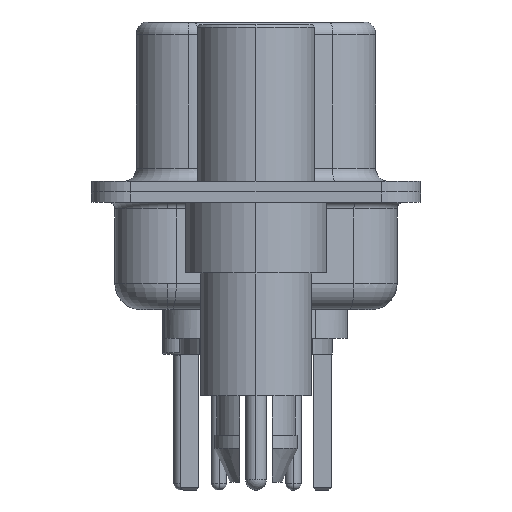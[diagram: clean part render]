
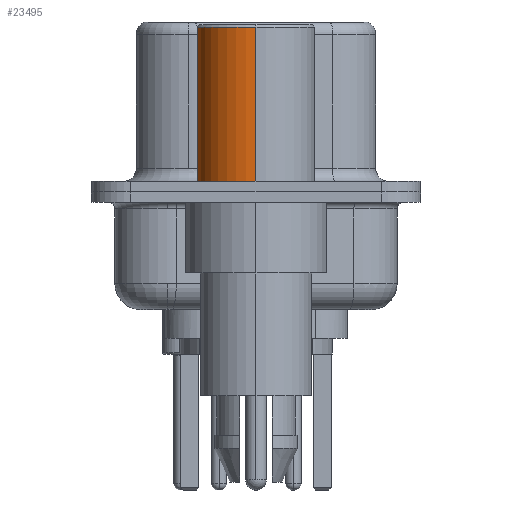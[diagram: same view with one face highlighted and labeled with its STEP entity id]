
A CAD part, left-side view. The second image highlights one B-rep face of the part: STEP entity #23495.
In plain terms, the highlighted cylindrical face has radius 2.25 mm (diameter 4.5 mm), a partial arc.
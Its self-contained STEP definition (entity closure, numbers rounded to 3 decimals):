
#470 = FACE_OUTER_BOUND ( 'NONE', #22428, .T. ) ;
#555 = DIRECTION ( 'NONE',  ( 0., 0., 1. ) ) ;
#798 = CARTESIAN_POINT ( 'NONE',  ( 0., 0., 0.4 ) ) ;
#839 = DIRECTION ( 'NONE',  ( 1., 0., 0. ) ) ;
#1047 = LINE ( 'NONE', #11443, #3647 ) ;
#1614 = CIRCLE ( 'NONE', #9624, 2.25 ) ;
#1945 = VECTOR ( 'NONE', #555, 1000. ) ;
#2211 = ORIENTED_EDGE ( 'NONE', *, *, #14536, .T. ) ;
#2398 = EDGE_CURVE ( 'NONE', #5247, #7590, #1614, .T. ) ;
#3647 = VECTOR ( 'NONE', #21915, 1000. ) ;
#3796 = ORIENTED_EDGE ( 'NONE', *, *, #12937, .F. ) ;
#4048 = AXIS2_PLACEMENT_3D ( 'NONE', #8427, #14633, #8522 ) ;
#5247 = VERTEX_POINT ( 'NONE', #15278 ) ;
#5337 = CYLINDRICAL_SURFACE ( 'NONE', #4048, 2.25 ) ;
#7590 = VERTEX_POINT ( 'NONE', #15728 ) ;
#7631 = CARTESIAN_POINT ( 'NONE',  ( -2.25, 0., 0.4 ) ) ;
#7761 = LINE ( 'NONE', #19326, #1945 ) ;
#8427 = CARTESIAN_POINT ( 'NONE',  ( 0., 0., 0.581 ) ) ;
#8464 = VERTEX_POINT ( 'NONE', #18188 ) ;
#8522 = DIRECTION ( 'NONE',  ( 1., 0., 0. ) ) ;
#9273 = ORIENTED_EDGE ( 'NONE', *, *, #2398, .F. ) ;
#9369 = VERTEX_POINT ( 'NONE', #7631 ) ;
#9624 = AXIS2_PLACEMENT_3D ( 'NONE', #15163, #23126, #839 ) ;
#11443 = CARTESIAN_POINT ( 'NONE',  ( 2.25, 0., 0.581 ) ) ;
#12937 = EDGE_CURVE ( 'NONE', #8464, #5247, #1047, .T. ) ;
#13337 = DIRECTION ( 'NONE',  ( 1., 0., 0. ) ) ;
#14536 = EDGE_CURVE ( 'NONE', #9369, #7590, #7761, .T. ) ;
#14623 = AXIS2_PLACEMENT_3D ( 'NONE', #798, #17398, #13337 ) ;
#14633 = DIRECTION ( 'NONE',  ( 0., 0., 1. ) ) ;
#15163 = CARTESIAN_POINT ( 'NONE',  ( 0., 0., 6.3 ) ) ;
#15278 = CARTESIAN_POINT ( 'NONE',  ( 2.25, 0., 6.3 ) ) ;
#15728 = CARTESIAN_POINT ( 'NONE',  ( -2.25, 0., 6.3 ) ) ;
#17398 = DIRECTION ( 'NONE',  ( 0., 0., 1. ) ) ;
#17486 = CIRCLE ( 'NONE', #14623, 2.25 ) ;
#18188 = CARTESIAN_POINT ( 'NONE',  ( 2.25, 0., 0.4 ) ) ;
#19326 = CARTESIAN_POINT ( 'NONE',  ( -2.25, 0., 0.581 ) ) ;
#21915 = DIRECTION ( 'NONE',  ( 0., 0., 1. ) ) ;
#22018 = ORIENTED_EDGE ( 'NONE', *, *, #25477, .T. ) ;
#22428 = EDGE_LOOP ( 'NONE', ( #22018, #2211, #9273, #3796 ) ) ;
#23126 = DIRECTION ( 'NONE',  ( 0., 0., 1. ) ) ;
#23495 = ADVANCED_FACE ( 'NONE', ( #470 ), #5337, .T. ) ;
#25477 = EDGE_CURVE ( 'NONE', #8464, #9369, #17486, .T. ) ;
